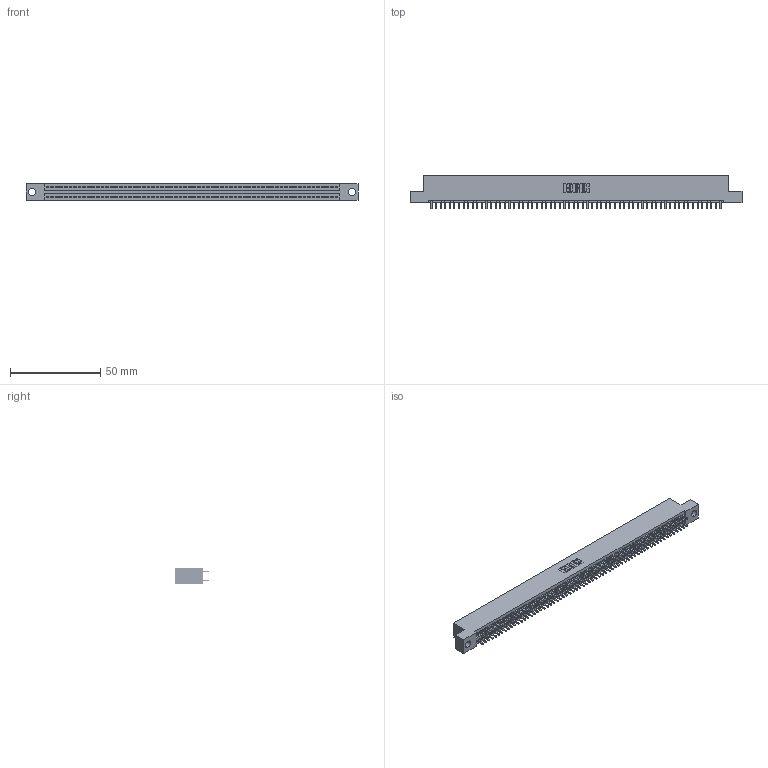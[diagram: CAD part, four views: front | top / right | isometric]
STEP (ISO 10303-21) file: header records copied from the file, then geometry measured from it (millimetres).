
FILE_DESCRIPTION (( 'STEP AP203' ), '1' );
FILE_NAME ('345-128-521-204.STEP', '2021-05-25T19:39:01', ( '' ), ( '' ), 'SwSTEP 2.0', 'SolidWorks 2020', '' );
FILE_SCHEMA (( 'CONFIG_CONTROL_DESIGN' ));
Length unit declared in the file: inch
Products named in the file (3): 345-128-521-204; 345-292-001_345-293-121; 345 Part_Flush Mounting Lugs - 0.156 Dia-TI
Assembly tree (129 placements, depth 2):
  345-128-521-204
    345 Part_Flush Mounting Lugs - 0.156 Dia-TI
    345-292-001_345-293-121  x128
Bounding box: 183.77 x 18.72 x 9.4 mm (x, y, z)
Volume: 17897.5 mm3; surface area: 26393.2 mm2
Topology: 129 solids, 129 shells, 6540 faces, 19449 edges, 12794 vertices
Faces by surface type: plane 4318, cylinder 2222
Entity records: 47691 total; most frequent: CARTESIAN_POINT 7978, ORIENTED_EDGE 7910, DIRECTION 7007, EDGE_CURVE 3955, VECTOR 3567, LINE 3567, VERTEX_POINT 2634, AXIS2_PLACEMENT_3D 1720
